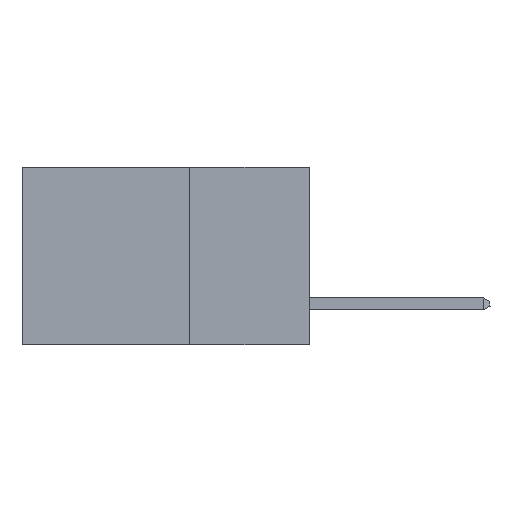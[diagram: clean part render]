
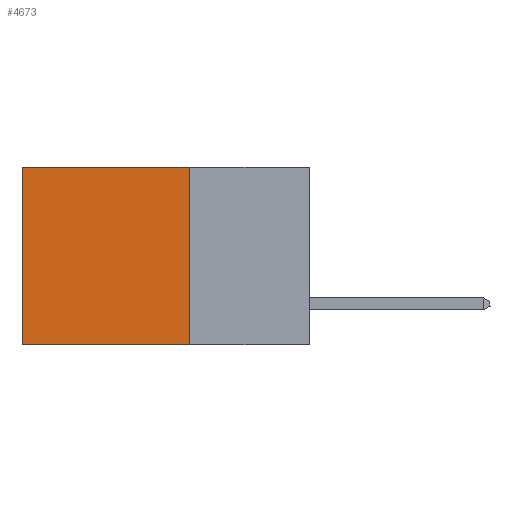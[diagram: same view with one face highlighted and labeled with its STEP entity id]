
A CAD part, left-side view. The second image highlights one B-rep face of the part: STEP entity #4673.
In plain terms, the highlighted planar face has unit normal (-1, 0, 0).
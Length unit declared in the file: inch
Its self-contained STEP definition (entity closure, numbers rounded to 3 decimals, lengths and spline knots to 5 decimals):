
#98 = CARTESIAN_POINT ( 'NONE',  ( 0.2875, 0.6, 0. ) ) ;
#781 = VERTEX_POINT ( 'NONE', #6402 ) ;
#837 = VECTOR ( 'NONE', #19834, 39.37008 ) ;
#1281 = CARTESIAN_POINT ( 'NONE',  ( 0.2875, 0.25, 0. ) ) ;
#4673 = ADVANCED_FACE ( 'NONE', ( #17092 ), #17598, .F. ) ;
#5071 = CARTESIAN_POINT ( 'NONE',  ( 0.2875, 0.25, 0. ) ) ;
#5465 = EDGE_LOOP ( 'NONE', ( #38021, #15951, #25282, #8437 ) ) ;
#6402 = CARTESIAN_POINT ( 'NONE',  ( 0.2875, 0.6, -0.37 ) ) ;
#8437 = ORIENTED_EDGE ( 'NONE', *, *, #21952, .T. ) ;
#8717 = DIRECTION ( 'NONE',  ( 0., 1., 0. ) ) ;
#8950 = CARTESIAN_POINT ( 'NONE',  ( 0.2875, 0.25, 0. ) ) ;
#12803 = LINE ( 'NONE', #1281, #33777 ) ;
#14015 = DIRECTION ( 'NONE',  ( 0., 0., -1. ) ) ;
#14058 = DIRECTION ( 'NONE',  ( 0., 1., 0. ) ) ;
#15951 = ORIENTED_EDGE ( 'NONE', *, *, #28921, .F. ) ;
#17092 = FACE_OUTER_BOUND ( 'NONE', #5465, .T. ) ;
#17598 = PLANE ( 'NONE',  #50321 ) ;
#17648 = CARTESIAN_POINT ( 'NONE',  ( 0.2875, 0.25, -0.37 ) ) ;
#18883 = EDGE_CURVE ( 'NONE', #42824, #22174, #27746, .T. ) ;
#19611 = LINE ( 'NONE', #39319, #49573 ) ;
#19834 = DIRECTION ( 'NONE',  ( 0., 0., -1. ) ) ;
#20935 = DIRECTION ( 'NONE',  ( 1., 0., 0. ) ) ;
#21952 = EDGE_CURVE ( 'NONE', #42824, #36758, #12803, .T. ) ;
#22174 = VERTEX_POINT ( 'NONE', #30162 ) ;
#23155 = CARTESIAN_POINT ( 'NONE',  ( 0.2875, 0.25, 0. ) ) ;
#23480 = VECTOR ( 'NONE', #14058, 39.37008 ) ;
#25282 = ORIENTED_EDGE ( 'NONE', *, *, #18883, .F. ) ;
#25367 = EDGE_CURVE ( 'NONE', #36758, #781, #19611, .T. ) ;
#27746 = LINE ( 'NONE', #23155, #837 ) ;
#28921 = EDGE_CURVE ( 'NONE', #22174, #781, #48355, .T. ) ;
#30162 = CARTESIAN_POINT ( 'NONE',  ( 0.2875, 0.25, -0.37 ) ) ;
#33777 = VECTOR ( 'NONE', #8717, 39.37008 ) ;
#34710 = DIRECTION ( 'NONE',  ( 0., 0., -1. ) ) ;
#36758 = VERTEX_POINT ( 'NONE', #98 ) ;
#38021 = ORIENTED_EDGE ( 'NONE', *, *, #25367, .T. ) ;
#39319 = CARTESIAN_POINT ( 'NONE',  ( 0.2875, 0.6, 0. ) ) ;
#42824 = VERTEX_POINT ( 'NONE', #8950 ) ;
#48355 = LINE ( 'NONE', #17648, #23480 ) ;
#49573 = VECTOR ( 'NONE', #34710, 39.37008 ) ;
#50321 = AXIS2_PLACEMENT_3D ( 'NONE', #5071, #20935, #14015 ) ;
